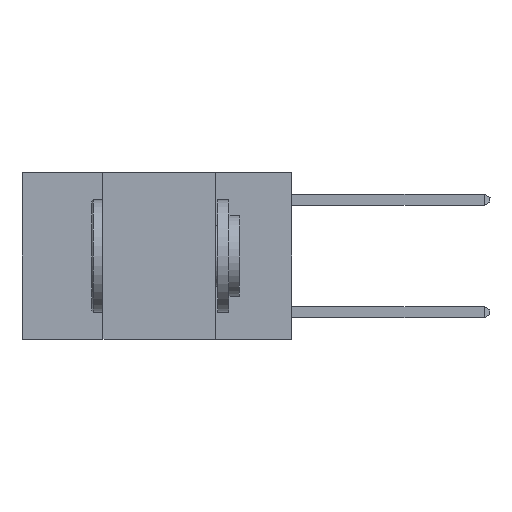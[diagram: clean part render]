
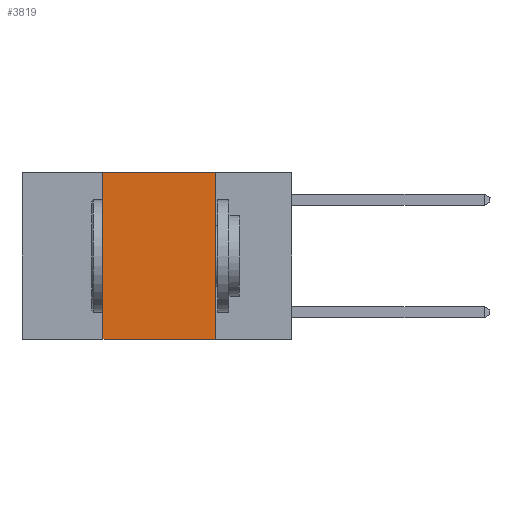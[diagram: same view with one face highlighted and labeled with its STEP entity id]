
A CAD part, left-side view. The second image highlights one B-rep face of the part: STEP entity #3819.
In plain terms, the highlighted planar face has unit normal (-1, 0, 0).
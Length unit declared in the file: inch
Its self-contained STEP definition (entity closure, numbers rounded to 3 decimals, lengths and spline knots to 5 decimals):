
#817 = VECTOR ( 'NONE', #4993, 39.37008 ) ;
#824 = ORIENTED_EDGE ( 'NONE', *, *, #9529, .F. ) ;
#895 = CARTESIAN_POINT ( 'NONE',  ( 0., 0.42, 0. ) ) ;
#1012 = CARTESIAN_POINT ( 'NONE',  ( 0., 0.42, 0. ) ) ;
#1915 = LINE ( 'NONE', #1012, #10390 ) ;
#2222 = CARTESIAN_POINT ( 'NONE',  ( 0., 0.17, 0. ) ) ;
#2702 = EDGE_CURVE ( 'NONE', #5077, #4998, #7489, .T. ) ;
#2812 = CARTESIAN_POINT ( 'NONE',  ( 0., 0.6, -0.37 ) ) ;
#3438 = PLANE ( 'NONE',  #6671 ) ;
#3465 = CARTESIAN_POINT ( 'NONE',  ( 0., 0.42, -0.37 ) ) ;
#3542 = DIRECTION ( 'NONE',  ( 0., 0., 1. ) ) ;
#3819 = ADVANCED_FACE ( 'NONE', ( #6852 ), #3438, .F. ) ;
#4306 = DIRECTION ( 'NONE',  ( 1., 0., 0. ) ) ;
#4506 = EDGE_CURVE ( 'NONE', #7501, #4998, #9176, .T. ) ;
#4690 = CARTESIAN_POINT ( 'NONE',  ( 0., 0.17, -0.37 ) ) ;
#4993 = DIRECTION ( 'NONE',  ( 0., 0., -1. ) ) ;
#4998 = VERTEX_POINT ( 'NONE', #4690 ) ;
#5077 = VERTEX_POINT ( 'NONE', #2222 ) ;
#5091 = DIRECTION ( 'NONE',  ( 0., -1., 0. ) ) ;
#5917 = CARTESIAN_POINT ( 'NONE',  ( 0., 0.6, 0. ) ) ;
#5992 = VECTOR ( 'NONE', #5091, 39.37008 ) ;
#6306 = CARTESIAN_POINT ( 'NONE',  ( 0., 0.17, 0. ) ) ;
#6671 = AXIS2_PLACEMENT_3D ( 'NONE', #9153, #4306, #9938 ) ;
#6852 = FACE_OUTER_BOUND ( 'NONE', #10611, .T. ) ;
#7089 = VECTOR ( 'NONE', #7790, 39.37008 ) ;
#7262 = ORIENTED_EDGE ( 'NONE', *, *, #2702, .F. ) ;
#7489 = LINE ( 'NONE', #6306, #817 ) ;
#7497 = ORIENTED_EDGE ( 'NONE', *, *, #7589, .F. ) ;
#7501 = VERTEX_POINT ( 'NONE', #3465 ) ;
#7589 = EDGE_CURVE ( 'NONE', #7501, #10281, #1915, .T. ) ;
#7790 = DIRECTION ( 'NONE',  ( 0., -1., 0. ) ) ;
#8380 = LINE ( 'NONE', #5917, #5992 ) ;
#9153 = CARTESIAN_POINT ( 'NONE',  ( 0., 0.6, 0. ) ) ;
#9176 = LINE ( 'NONE', #2812, #7089 ) ;
#9529 = EDGE_CURVE ( 'NONE', #10281, #5077, #8380, .T. ) ;
#9604 = ORIENTED_EDGE ( 'NONE', *, *, #4506, .T. ) ;
#9938 = DIRECTION ( 'NONE',  ( 0., 0., -1. ) ) ;
#10281 = VERTEX_POINT ( 'NONE', #895 ) ;
#10390 = VECTOR ( 'NONE', #3542, 39.37008 ) ;
#10611 = EDGE_LOOP ( 'NONE', ( #7262, #824, #7497, #9604 ) ) ;
